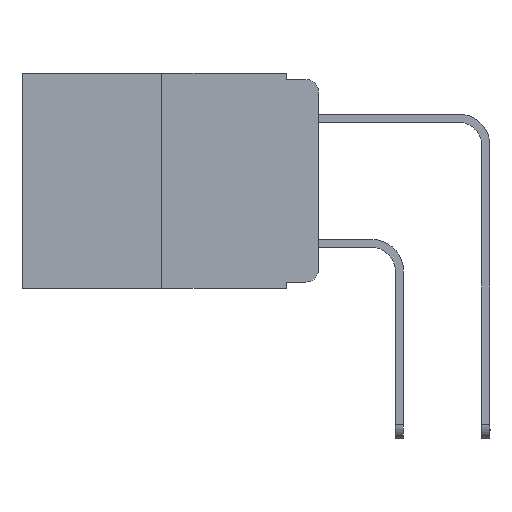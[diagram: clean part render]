
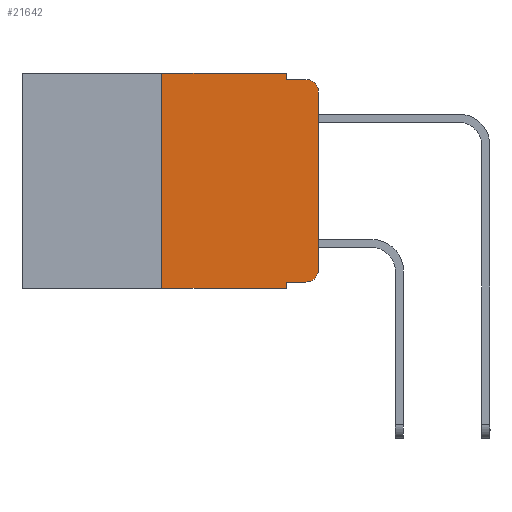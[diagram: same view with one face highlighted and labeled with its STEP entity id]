
A CAD part, left-side view. The second image highlights one B-rep face of the part: STEP entity #21642.
In plain terms, the highlighted planar face has unit normal (-1, 0, 0).
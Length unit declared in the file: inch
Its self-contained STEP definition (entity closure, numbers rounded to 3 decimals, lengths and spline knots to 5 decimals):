
#19 = DIRECTION ( 'NONE',  ( 0., 0., -1. ) ) ;
#726 = LINE ( 'NONE', #20154, #1815 ) ;
#1498 = VERTEX_POINT ( 'NONE', #21198 ) ;
#1675 = EDGE_CURVE ( 'NONE', #5864, #15745, #726, .T. ) ;
#1696 = VERTEX_POINT ( 'NONE', #16579 ) ;
#1725 = VERTEX_POINT ( 'NONE', #8358 ) ;
#1815 = VECTOR ( 'NONE', #10076, 39.37008 ) ;
#2137 = LINE ( 'NONE', #7227, #19074 ) ;
#2471 = EDGE_LOOP ( 'NONE', ( #7407, #12300, #13012, #2888, #20934, #5505, #3129, #7627, #17120, #20180 ) ) ;
#2586 = VERTEX_POINT ( 'NONE', #5541 ) ;
#2757 = CARTESIAN_POINT ( 'NONE',  ( 0., 0., 0. ) ) ;
#2888 = ORIENTED_EDGE ( 'NONE', *, *, #20161, .F. ) ;
#3129 = ORIENTED_EDGE ( 'NONE', *, *, #16951, .T. ) ;
#3222 = EDGE_CURVE ( 'NONE', #1725, #5864, #16297, .T. ) ;
#3363 = CARTESIAN_POINT ( 'NONE',  ( 0., 0., -0.313 ) ) ;
#3370 = AXIS2_PLACEMENT_3D ( 'NONE', #5436, #20314, #3524 ) ;
#3479 = VERTEX_POINT ( 'NONE', #9792 ) ;
#3524 = DIRECTION ( 'NONE',  ( 0., 0., -1. ) ) ;
#3544 = LINE ( 'NONE', #13331, #7535 ) ;
#3913 = CARTESIAN_POINT ( 'NONE',  ( 0., 0.051, -0.01 ) ) ;
#4654 = AXIS2_PLACEMENT_3D ( 'NONE', #4763, #21436, #13183 ) ;
#4763 = CARTESIAN_POINT ( 'NONE',  ( 0., 0.02, -0.03 ) ) ;
#4783 = CARTESIAN_POINT ( 'NONE',  ( 0., 0.02, -0.313 ) ) ;
#4938 = DIRECTION ( 'NONE',  ( -1., 0., 0. ) ) ;
#5436 = CARTESIAN_POINT ( 'NONE',  ( 0., 0.473, 0. ) ) ;
#5505 = ORIENTED_EDGE ( 'NONE', *, *, #3222, .F. ) ;
#5541 = CARTESIAN_POINT ( 'NONE',  ( 0., 0.051, -0.01 ) ) ;
#5864 = VERTEX_POINT ( 'NONE', #7742 ) ;
#5991 = LINE ( 'NONE', #18764, #13718 ) ;
#7113 = VECTOR ( 'NONE', #16064, 39.37008 ) ;
#7227 = CARTESIAN_POINT ( 'NONE',  ( 0., 0.473, -0.343 ) ) ;
#7407 = ORIENTED_EDGE ( 'NONE', *, *, #7881, .T. ) ;
#7535 = VECTOR ( 'NONE', #19, 39.37008 ) ;
#7611 = CARTESIAN_POINT ( 'NONE',  ( 0., 0.25, 0. ) ) ;
#7627 = ORIENTED_EDGE ( 'NONE', *, *, #8963, .F. ) ;
#7677 = FACE_OUTER_BOUND ( 'NONE', #2471, .T. ) ;
#7742 = CARTESIAN_POINT ( 'NONE',  ( 0., 0.25, 0. ) ) ;
#7881 = EDGE_CURVE ( 'NONE', #9600, #1696, #16095, .T. ) ;
#8042 = LINE ( 'NONE', #3913, #10438 ) ;
#8358 = CARTESIAN_POINT ( 'NONE',  ( 0., 0.25, -0.343 ) ) ;
#8734 = EDGE_CURVE ( 'NONE', #3479, #12034, #16003, .T. ) ;
#8963 = EDGE_CURVE ( 'NONE', #3479, #1498, #3544, .T. ) ;
#9426 = VECTOR ( 'NONE', #11237, 39.37008 ) ;
#9600 = VERTEX_POINT ( 'NONE', #3363 ) ;
#9792 = CARTESIAN_POINT ( 'NONE',  ( 0., 0.051, -0.333 ) ) ;
#9923 = EDGE_CURVE ( 'NONE', #2586, #18710, #8042, .T. ) ;
#10076 = DIRECTION ( 'NONE',  ( 0., -1., 0. ) ) ;
#10438 = VECTOR ( 'NONE', #12475, 39.37008 ) ;
#11237 = DIRECTION ( 'NONE',  ( 0., -1., 0. ) ) ;
#12034 = VERTEX_POINT ( 'NONE', #19215 ) ;
#12080 = DIRECTION ( 'NONE',  ( 0., 0., -1. ) ) ;
#12117 = VECTOR ( 'NONE', #19483, 39.37008 ) ;
#12300 = ORIENTED_EDGE ( 'NONE', *, *, #16718, .T. ) ;
#12348 = DIRECTION ( 'NONE',  ( 0., -1., 0. ) ) ;
#12475 = DIRECTION ( 'NONE',  ( 0., -1., 0. ) ) ;
#13012 = ORIENTED_EDGE ( 'NONE', *, *, #9923, .F. ) ;
#13183 = DIRECTION ( 'NONE',  ( 0., 0., -1. ) ) ;
#13331 = CARTESIAN_POINT ( 'NONE',  ( 0., 0.051, 0. ) ) ;
#13474 = AXIS2_PLACEMENT_3D ( 'NONE', #4783, #4938, #21763 ) ;
#13718 = VECTOR ( 'NONE', #12080, 39.37008 ) ;
#13841 = EDGE_CURVE ( 'NONE', #12034, #9600, #15775, .T. ) ;
#15389 = PLANE ( 'NONE',  #3370 ) ;
#15745 = VERTEX_POINT ( 'NONE', #19008 ) ;
#15775 = CIRCLE ( 'NONE', #13474, 0.02 ) ;
#16003 = LINE ( 'NONE', #21257, #9426 ) ;
#16064 = DIRECTION ( 'NONE',  ( 0., 0., 1. ) ) ;
#16095 = LINE ( 'NONE', #2757, #7113 ) ;
#16297 = LINE ( 'NONE', #7611, #12117 ) ;
#16443 = CIRCLE ( 'NONE', #4654, 0.02 ) ;
#16579 = CARTESIAN_POINT ( 'NONE',  ( 0., 0., -0.03 ) ) ;
#16718 = EDGE_CURVE ( 'NONE', #1696, #18710, #16443, .T. ) ;
#16951 = EDGE_CURVE ( 'NONE', #1725, #1498, #2137, .T. ) ;
#17120 = ORIENTED_EDGE ( 'NONE', *, *, #8734, .T. ) ;
#18710 = VERTEX_POINT ( 'NONE', #21871 ) ;
#18764 = CARTESIAN_POINT ( 'NONE',  ( 0., 0.051, 0. ) ) ;
#19008 = CARTESIAN_POINT ( 'NONE',  ( 0., 0.051, 0. ) ) ;
#19074 = VECTOR ( 'NONE', #12348, 39.37008 ) ;
#19215 = CARTESIAN_POINT ( 'NONE',  ( 0., 0.02, -0.333 ) ) ;
#19483 = DIRECTION ( 'NONE',  ( 0., 0., 1. ) ) ;
#20154 = CARTESIAN_POINT ( 'NONE',  ( 0., 0.473, 0. ) ) ;
#20161 = EDGE_CURVE ( 'NONE', #15745, #2586, #5991, .T. ) ;
#20180 = ORIENTED_EDGE ( 'NONE', *, *, #13841, .T. ) ;
#20314 = DIRECTION ( 'NONE',  ( 1., 0., 0. ) ) ;
#20934 = ORIENTED_EDGE ( 'NONE', *, *, #1675, .F. ) ;
#21198 = CARTESIAN_POINT ( 'NONE',  ( 0., 0.051, -0.343 ) ) ;
#21257 = CARTESIAN_POINT ( 'NONE',  ( 0., 0.051, -0.333 ) ) ;
#21436 = DIRECTION ( 'NONE',  ( -1., 0., 0. ) ) ;
#21642 = ADVANCED_FACE ( 'NONE', ( #7677 ), #15389, .F. ) ;
#21763 = DIRECTION ( 'NONE',  ( 0., 0., -1. ) ) ;
#21871 = CARTESIAN_POINT ( 'NONE',  ( 0., 0.02, -0.01 ) ) ;
